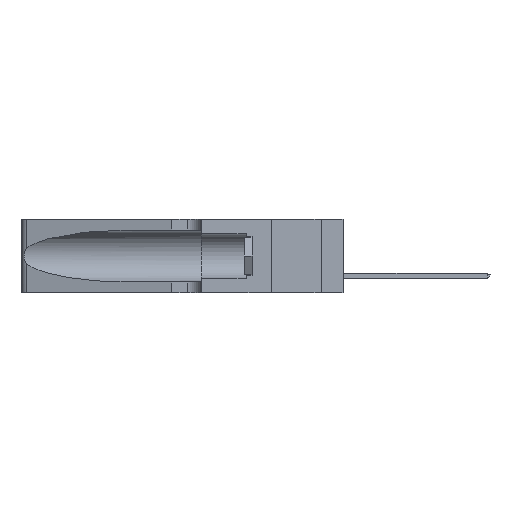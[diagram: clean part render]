
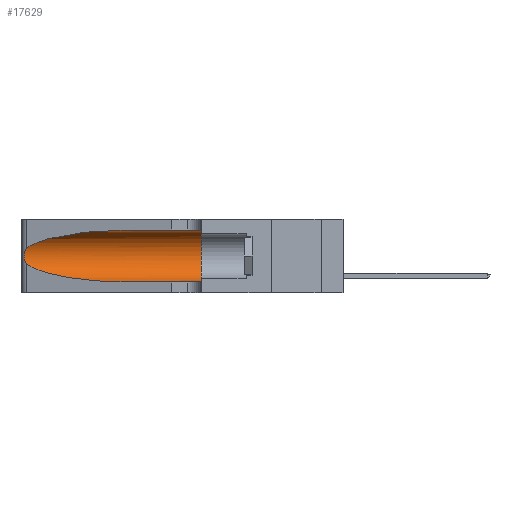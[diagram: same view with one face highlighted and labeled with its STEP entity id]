
A CAD part, left-side view. The second image highlights one B-rep face of the part: STEP entity #17629.
In plain terms, the highlighted cylindrical face has radius 3.308 mm (diameter 6.617 mm), a partial arc.
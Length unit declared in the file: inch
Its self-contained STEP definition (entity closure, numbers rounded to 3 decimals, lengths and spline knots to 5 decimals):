
#1033 = VERTEX_POINT ( 'NONE', #26157 ) ;
#1060 = EDGE_CURVE ( 'NONE', #15805, #21998, #9107, .T. ) ;
#1397 = CARTESIAN_POINT ( 'NONE',  ( 0.1305, 0.72297, 0.31525 ) ) ;
#2113 = CARTESIAN_POINT ( 'NONE',  ( 0.25639, 1.23186, 0.15144 ) ) ;
#2293 = EDGE_CURVE ( 'NONE', #21084, #1033, #23046, .T. ) ;
#2315 = CARTESIAN_POINT ( 'NONE',  ( 0.25487, 1.22718, 0.14631 ) ) ;
#2348 = DIRECTION ( 'NONE',  ( 0., -1., 0. ) ) ;
#3475 = CARTESIAN_POINT ( 'NONE',  ( 0.1305, 0.35, 0.185 ) ) ;
#3703 = CARTESIAN_POINT ( 'NONE',  ( 0.1305, 0.72297, 0.31525 ) ) ;
#5187 = DIRECTION ( 'NONE',  ( 0., 0., -1. ) ) ;
#5322 = DIRECTION ( 'NONE',  ( 0., -1., 0. ) ) ;
#5878 = DIRECTION ( 'NONE',  ( 0., 1., 0. ) ) ;
#5976 = DIRECTION ( 'NONE',  ( 0., 0., 1. ) ) ;
#6009 = ORIENTED_EDGE ( 'NONE', *, *, #18718, .T. ) ;
#6675 = CARTESIAN_POINT ( 'NONE',  ( 0.26075, 1.23896, 0.178 ) ) ;
#6973 = CARTESIAN_POINT ( 'NONE',  ( 0.25856, 1.23593, 0.16098 ) ) ;
#6979 = ORIENTED_EDGE ( 'NONE', *, *, #1060, .T. ) ;
#7085 = EDGE_CURVE ( 'NONE', #8162, #21998, #12101, .T. ) ;
#7234 = VECTOR ( 'NONE', #5322, 39.37008 ) ;
#7239 = CARTESIAN_POINT ( 'NONE',  ( 0.25555, 1.22993, 0.14849 ) ) ;
#7923 = CARTESIAN_POINT ( 'NONE',  ( 0.25487, 1.22718, 0.14631 ) ) ;
#8162 = VERTEX_POINT ( 'NONE', #13686 ) ;
#9107 = LINE ( 'NONE', #14000, #12786 ) ;
#9702 = ORIENTED_EDGE ( 'NONE', *, *, #16677, .T. ) ;
#9933 = CARTESIAN_POINT ( 'NONE',  ( 0.1305, 1.61858, 0.31525 ) ) ;
#10695 = CYLINDRICAL_SURFACE ( 'NONE', #13858, 0.13025 ) ;
#11399 = CARTESIAN_POINT ( 'NONE',  ( 0.26075, 1.23896, 0.19203 ) ) ;
#12101 = CIRCLE ( 'NONE', #19017, 0.13025 ) ;
#12603 = ORIENTED_EDGE ( 'NONE', *, *, #7085, .F. ) ;
#12786 = VECTOR ( 'NONE', #2348, 39.37008 ) ;
#12878 = ORIENTED_EDGE ( 'NONE', *, *, #19807, .F. ) ;
#13686 = CARTESIAN_POINT ( 'NONE',  ( 0.1305, 0.35, 0.31525 ) ) ;
#13858 = AXIS2_PLACEMENT_3D ( 'NONE', #16940, #19323, #5187 ) ;
#14000 = CARTESIAN_POINT ( 'NONE',  ( 0.1305, 1.61858, 0.05475 ) ) ;
#15805 = VERTEX_POINT ( 'NONE', #28023 ) ;
#16258 = ORIENTED_EDGE ( 'NONE', *, *, #2293, .T. ) ;
#16262 = CARTESIAN_POINT ( 'NONE',  ( 0.25789, 1.23486, 0.15765 ) ) ;
#16462 = CARTESIAN_POINT ( 'NONE',  ( 0.2373, 1.15595, 0.28018 ) ) ;
#16677 = EDGE_CURVE ( 'NONE', #20611, #21084, #17531, .T. ) ;
#16940 = CARTESIAN_POINT ( 'NONE',  ( 0.1305, 1.61858, 0.185 ) ) ;
#17531 =( BOUNDED_CURVE ( )  B_SPLINE_CURVE ( 3, ( #1397, #17944, #16462, #28129 ),
 .UNSPECIFIED., .F., .F. ) 
 B_SPLINE_CURVE_WITH_KNOTS ( ( 4, 4 ),
 ( 1.5708, 2.84003 ),
 .UNSPECIFIED. ) 
 CURVE ( )  GEOMETRIC_REPRESENTATION_ITEM ( )  RATIONAL_B_SPLINE_CURVE ( ( 1., 0.87, 0.87, 1. ) ) 
 REPRESENTATION_ITEM ( '' )  );
#17629 = ADVANCED_FACE ( 'NONE', ( #23657 ), #10695, .F. ) ;
#17944 = CARTESIAN_POINT ( 'NONE',  ( 0.18966, 0.96281, 0.31525 ) ) ;
#18718 = EDGE_CURVE ( 'NONE', #1033, #15805, #20769, .T. ) ;
#18746 = CARTESIAN_POINT ( 'NONE',  ( 0.25555, 1.22994, 0.2215 ) ) ;
#19017 = AXIS2_PLACEMENT_3D ( 'NONE', #3475, #5878, #5976 ) ;
#19323 = DIRECTION ( 'NONE',  ( 0., -1., 0. ) ) ;
#19605 = CARTESIAN_POINT ( 'NONE',  ( 0.1305, 0.72297, 0.05475 ) ) ;
#19806 = LINE ( 'NONE', #9933, #7234 ) ;
#19807 = EDGE_CURVE ( 'NONE', #20611, #8162, #19806, .T. ) ;
#20611 = VERTEX_POINT ( 'NONE', #3703 ) ;
#20699 = CARTESIAN_POINT ( 'NONE',  ( 0.25487, 1.22718, 0.22369 ) ) ;
#20769 =( BOUNDED_CURVE ( )  B_SPLINE_CURVE ( 3, ( #7923, #24328, #24135, #19605 ),
 .UNSPECIFIED., .F., .F. ) 
 B_SPLINE_CURVE_WITH_KNOTS ( ( 4, 4 ),
 ( 3.44316, 4.71239 ),
 .UNSPECIFIED. ) 
 CURVE ( )  GEOMETRIC_REPRESENTATION_ITEM ( )  RATIONAL_B_SPLINE_CURVE ( ( 1., 0.87, 0.87, 1. ) ) 
 REPRESENTATION_ITEM ( '' )  );
#20809 = CARTESIAN_POINT ( 'NONE',  ( 0.26018, 1.23835, 0.19895 ) ) ;
#21084 = VERTEX_POINT ( 'NONE', #25310 ) ;
#21097 = CARTESIAN_POINT ( 'NONE',  ( 0.25854, 1.2359, 0.20912 ) ) ;
#21998 = VERTEX_POINT ( 'NONE', #30264 ) ;
#23046 = B_SPLINE_CURVE_WITH_KNOTS ( 'NONE', 3,
 ( #20699, #18746, #23087, #25853, #21097, #20809, #11399, #6675, #30422, #6973, #16262, #2113, #7239, #2315 ),
 .UNSPECIFIED., .F., .F.,
 ( 4, 2, 2, 2, 2, 2, 4 ),
 ( 0., 0.00027, 0.00053, 0.00107, 0.0016, 0.00187, 0.00214 ),
 .UNSPECIFIED. ) ;
#23087 = CARTESIAN_POINT ( 'NONE',  ( 0.25639, 1.23184, 0.21858 ) ) ;
#23657 = FACE_OUTER_BOUND ( 'NONE', #24344, .T. ) ;
#24135 = CARTESIAN_POINT ( 'NONE',  ( 0.18966, 0.96281, 0.05475 ) ) ;
#24328 = CARTESIAN_POINT ( 'NONE',  ( 0.2373, 1.15595, 0.08982 ) ) ;
#24344 = EDGE_LOOP ( 'NONE', ( #9702, #16258, #6009, #6979, #12603, #12878 ) ) ;
#25310 = CARTESIAN_POINT ( 'NONE',  ( 0.25487, 1.22718, 0.22369 ) ) ;
#25853 = CARTESIAN_POINT ( 'NONE',  ( 0.25787, 1.23484, 0.2124 ) ) ;
#26157 = CARTESIAN_POINT ( 'NONE',  ( 0.25487, 1.22718, 0.14631 ) ) ;
#28023 = CARTESIAN_POINT ( 'NONE',  ( 0.1305, 0.72297, 0.05475 ) ) ;
#28129 = CARTESIAN_POINT ( 'NONE',  ( 0.25487, 1.22718, 0.22369 ) ) ;
#30264 = CARTESIAN_POINT ( 'NONE',  ( 0.1305, 0.35, 0.05475 ) ) ;
#30422 = CARTESIAN_POINT ( 'NONE',  ( 0.26017, 1.23833, 0.17102 ) ) ;
